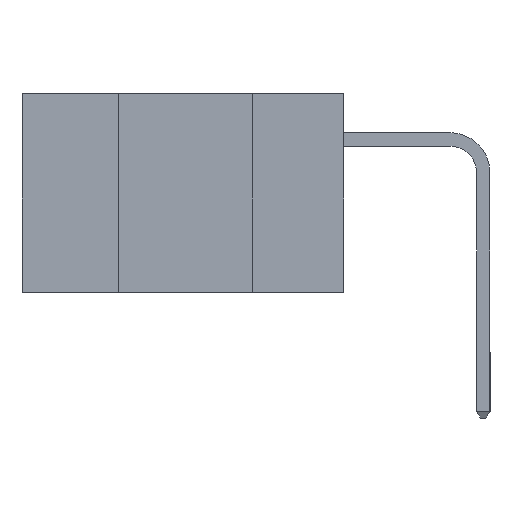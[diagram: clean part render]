
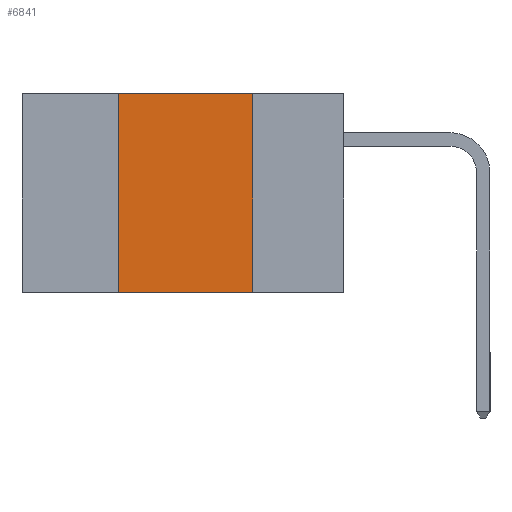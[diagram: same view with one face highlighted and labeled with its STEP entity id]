
A CAD part, left-side view. The second image highlights one B-rep face of the part: STEP entity #6841.
In plain terms, the highlighted planar face has unit normal (-1, 0, 0).
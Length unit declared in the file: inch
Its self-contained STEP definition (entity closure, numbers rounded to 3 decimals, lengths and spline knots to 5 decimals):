
#80 = CARTESIAN_POINT ( 'NONE',  ( 0., 0.17, -0.37 ) ) ;
#133 = VECTOR ( 'NONE', #14410, 39.37008 ) ;
#249 = VECTOR ( 'NONE', #13016, 39.37008 ) ;
#258 = CARTESIAN_POINT ( 'NONE',  ( 0., 0.17, 0. ) ) ;
#869 = LINE ( 'NONE', #5893, #10024 ) ;
#1422 = VERTEX_POINT ( 'NONE', #80 ) ;
#2028 = CARTESIAN_POINT ( 'NONE',  ( 0., 0.6, 0. ) ) ;
#2172 = CARTESIAN_POINT ( 'NONE',  ( 0., 0.17, 0. ) ) ;
#2293 = CARTESIAN_POINT ( 'NONE',  ( 0., 0.6, 0. ) ) ;
#2900 = CARTESIAN_POINT ( 'NONE',  ( 0., 0.42, -0.37 ) ) ;
#3198 = DIRECTION ( 'NONE',  ( 0., 0., -1. ) ) ;
#3352 = DIRECTION ( 'NONE',  ( 1., 0., 0. ) ) ;
#3414 = DIRECTION ( 'NONE',  ( 0., 0., 1. ) ) ;
#3666 = EDGE_CURVE ( 'NONE', #12685, #1422, #6041, .T. ) ;
#3952 = EDGE_CURVE ( 'NONE', #7554, #1422, #15264, .T. ) ;
#4916 = VERTEX_POINT ( 'NONE', #5144 ) ;
#4933 = VECTOR ( 'NONE', #10281, 39.37008 ) ;
#5144 = CARTESIAN_POINT ( 'NONE',  ( 0., 0.42, 0. ) ) ;
#5893 = CARTESIAN_POINT ( 'NONE',  ( 0., 0.42, 0. ) ) ;
#6041 = LINE ( 'NONE', #13535, #4933 ) ;
#6563 = LINE ( 'NONE', #2293, #249 ) ;
#6841 = ADVANCED_FACE ( 'NONE', ( #14199 ), #12852, .F. ) ;
#7554 = VERTEX_POINT ( 'NONE', #2172 ) ;
#7931 = ORIENTED_EDGE ( 'NONE', *, *, #9173, .F. ) ;
#9173 = EDGE_CURVE ( 'NONE', #12685, #4916, #869, .T. ) ;
#9495 = ORIENTED_EDGE ( 'NONE', *, *, #3666, .T. ) ;
#9558 = AXIS2_PLACEMENT_3D ( 'NONE', #2028, #3352, #3198 ) ;
#10024 = VECTOR ( 'NONE', #3414, 39.37008 ) ;
#10281 = DIRECTION ( 'NONE',  ( 0., -1., 0. ) ) ;
#11339 = ORIENTED_EDGE ( 'NONE', *, *, #14654, .F. ) ;
#12685 = VERTEX_POINT ( 'NONE', #2900 ) ;
#12852 = PLANE ( 'NONE',  #9558 ) ;
#13016 = DIRECTION ( 'NONE',  ( 0., -1., 0. ) ) ;
#13535 = CARTESIAN_POINT ( 'NONE',  ( 0., 0.6, -0.37 ) ) ;
#14199 = FACE_OUTER_BOUND ( 'NONE', #15092, .T. ) ;
#14410 = DIRECTION ( 'NONE',  ( 0., 0., -1. ) ) ;
#14654 = EDGE_CURVE ( 'NONE', #4916, #7554, #6563, .T. ) ;
#15092 = EDGE_LOOP ( 'NONE', ( #15234, #11339, #7931, #9495 ) ) ;
#15234 = ORIENTED_EDGE ( 'NONE', *, *, #3952, .F. ) ;
#15264 = LINE ( 'NONE', #258, #133 ) ;
